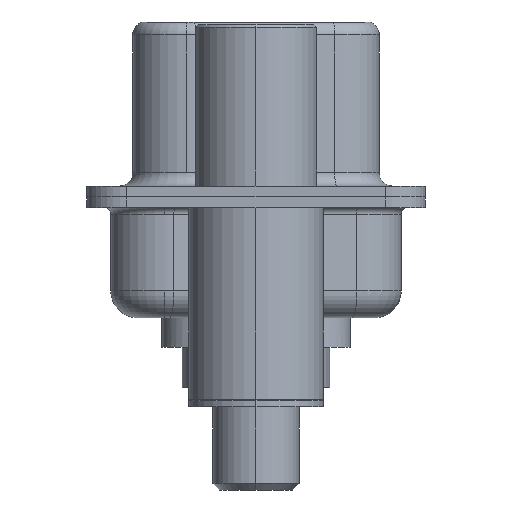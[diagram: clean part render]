
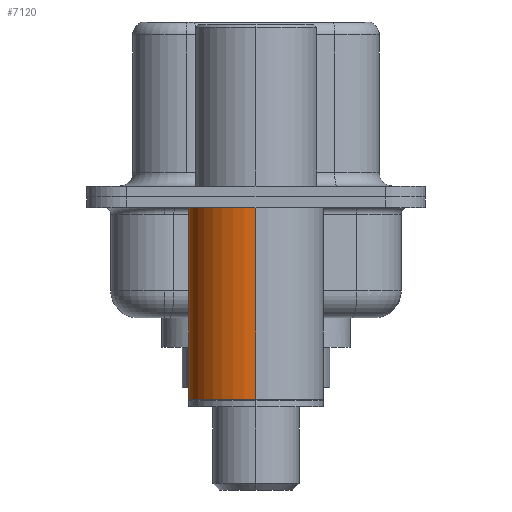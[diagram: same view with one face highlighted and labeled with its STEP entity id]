
A CAD part, left-side view. The second image highlights one B-rep face of the part: STEP entity #7120.
In plain terms, the highlighted cylindrical face has radius 2.5 mm (diameter 5 mm), a partial arc.
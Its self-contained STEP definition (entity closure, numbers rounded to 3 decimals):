
#537 = ORIENTED_EDGE ( 'NONE', *, *, #15031, .F. ) ;
#887 = CARTESIAN_POINT ( 'NONE',  ( -2.5, 0., 0.581 ) ) ;
#1852 = CARTESIAN_POINT ( 'NONE',  ( 2.5, 0., 0.581 ) ) ;
#2193 = CARTESIAN_POINT ( 'NONE',  ( 0., 0., -0.4 ) ) ;
#2287 = ORIENTED_EDGE ( 'NONE', *, *, #10642, .T. ) ;
#2791 = EDGE_CURVE ( 'NONE', #5678, #3959, #15840, .T. ) ;
#3459 = DIRECTION ( 'NONE',  ( 1., 0., 0. ) ) ;
#3563 = CYLINDRICAL_SURFACE ( 'NONE', #7229, 2.5 ) ;
#3722 = EDGE_CURVE ( 'NONE', #5678, #5661, #8643, .T. ) ;
#3959 = VERTEX_POINT ( 'NONE', #13288 ) ;
#4139 = ORIENTED_EDGE ( 'NONE', *, *, #3722, .T. ) ;
#5630 = AXIS2_PLACEMENT_3D ( 'NONE', #12236, #11371, #10013 ) ;
#5661 = VERTEX_POINT ( 'NONE', #8454 ) ;
#5678 = VERTEX_POINT ( 'NONE', #7037 ) ;
#6180 = CIRCLE ( 'NONE', #6191, 2.5 ) ;
#6191 = AXIS2_PLACEMENT_3D ( 'NONE', #2193, #10935, #3459 ) ;
#6263 = VECTOR ( 'NONE', #13435, 1000. ) ;
#7037 = CARTESIAN_POINT ( 'NONE',  ( 2.5, 0., -7.525 ) ) ;
#7048 = CARTESIAN_POINT ( 'NONE',  ( 0., 0., 0.581 ) ) ;
#7120 = ADVANCED_FACE ( 'NONE', ( #7586 ), #3563, .T. ) ;
#7131 = DIRECTION ( 'NONE',  ( 0., 0., 1. ) ) ;
#7229 = AXIS2_PLACEMENT_3D ( 'NONE', #7048, #8122, #8274 ) ;
#7586 = FACE_OUTER_BOUND ( 'NONE', #15564, .T. ) ;
#8122 = DIRECTION ( 'NONE',  ( 0., 0., 1. ) ) ;
#8274 = DIRECTION ( 'NONE',  ( 1., 0., 0. ) ) ;
#8454 = CARTESIAN_POINT ( 'NONE',  ( -2.5, 0., -7.525 ) ) ;
#8643 = CIRCLE ( 'NONE', #5630, 2.5 ) ;
#8793 = VERTEX_POINT ( 'NONE', #15606 ) ;
#10013 = DIRECTION ( 'NONE',  ( 1., 0., 0. ) ) ;
#10642 = EDGE_CURVE ( 'NONE', #5661, #8793, #12975, .T. ) ;
#10935 = DIRECTION ( 'NONE',  ( 0., 0., 1. ) ) ;
#11371 = DIRECTION ( 'NONE',  ( 0., 0., 1. ) ) ;
#12236 = CARTESIAN_POINT ( 'NONE',  ( 0., 0., -7.525 ) ) ;
#12658 = VECTOR ( 'NONE', #7131, 1000. ) ;
#12975 = LINE ( 'NONE', #887, #6263 ) ;
#13288 = CARTESIAN_POINT ( 'NONE',  ( 2.5, 0., -0.4 ) ) ;
#13435 = DIRECTION ( 'NONE',  ( 0., 0., 1. ) ) ;
#15031 = EDGE_CURVE ( 'NONE', #3959, #8793, #6180, .T. ) ;
#15543 = ORIENTED_EDGE ( 'NONE', *, *, #2791, .F. ) ;
#15564 = EDGE_LOOP ( 'NONE', ( #4139, #2287, #537, #15543 ) ) ;
#15606 = CARTESIAN_POINT ( 'NONE',  ( -2.5, 0., -0.4 ) ) ;
#15840 = LINE ( 'NONE', #1852, #12658 ) ;
